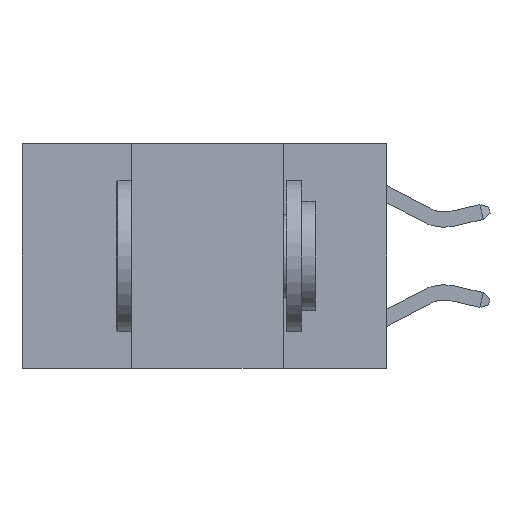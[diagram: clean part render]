
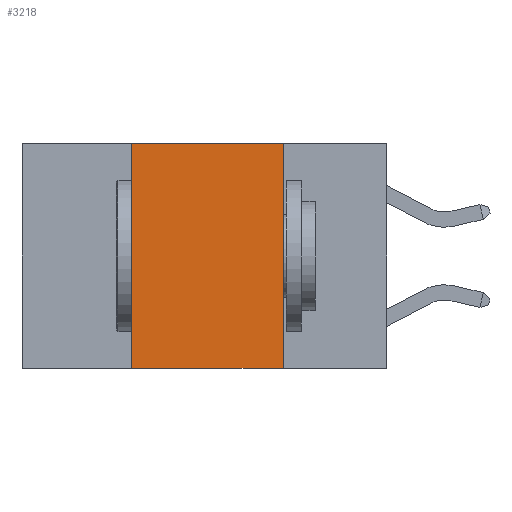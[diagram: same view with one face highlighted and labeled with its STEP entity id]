
A CAD part, left-side view. The second image highlights one B-rep face of the part: STEP entity #3218.
In plain terms, the highlighted planar face has unit normal (-1, 0, 0).
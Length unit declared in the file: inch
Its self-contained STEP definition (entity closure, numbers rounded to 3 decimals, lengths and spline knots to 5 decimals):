
#52 = DIRECTION ( 'NONE',  ( 1., 0., 0. ) ) ;
#83 = CARTESIAN_POINT ( 'NONE',  ( 0., 0.42, -0.37 ) ) ;
#806 = VERTEX_POINT ( 'NONE', #83 ) ;
#929 = VERTEX_POINT ( 'NONE', #12667 ) ;
#1819 = ORIENTED_EDGE ( 'NONE', *, *, #6716, .F. ) ;
#2478 = ORIENTED_EDGE ( 'NONE', *, *, #9090, .T. ) ;
#2516 = CARTESIAN_POINT ( 'NONE',  ( 0., 0.6, 0. ) ) ;
#3015 = DIRECTION ( 'NONE',  ( 0., 0., -1. ) ) ;
#3218 = ADVANCED_FACE ( 'NONE', ( #7715 ), #7903, .F. ) ;
#4309 = AXIS2_PLACEMENT_3D ( 'NONE', #4913, #52, #5985 ) ;
#4599 = DIRECTION ( 'NONE',  ( 0., -1., 0. ) ) ;
#4606 = CARTESIAN_POINT ( 'NONE',  ( 0., 0.6, -0.37 ) ) ;
#4913 = CARTESIAN_POINT ( 'NONE',  ( 0., 0.6, 0. ) ) ;
#5049 = VERTEX_POINT ( 'NONE', #6504 ) ;
#5470 = VECTOR ( 'NONE', #7691, 39.37008 ) ;
#5887 = LINE ( 'NONE', #2516, #11035 ) ;
#5985 = DIRECTION ( 'NONE',  ( 0., 0., -1. ) ) ;
#6270 = EDGE_CURVE ( 'NONE', #806, #10207, #7948, .T. ) ;
#6504 = CARTESIAN_POINT ( 'NONE',  ( 0., 0.17, 0. ) ) ;
#6660 = EDGE_LOOP ( 'NONE', ( #1819, #7339, #13161, #2478 ) ) ;
#6716 = EDGE_CURVE ( 'NONE', #5049, #929, #9691, .T. ) ;
#7280 = CARTESIAN_POINT ( 'NONE',  ( 0., 0.42, 0. ) ) ;
#7284 = VECTOR ( 'NONE', #3015, 39.37008 ) ;
#7339 = ORIENTED_EDGE ( 'NONE', *, *, #12444, .F. ) ;
#7691 = DIRECTION ( 'NONE',  ( 0., -1., 0. ) ) ;
#7715 = FACE_OUTER_BOUND ( 'NONE', #6660, .T. ) ;
#7903 = PLANE ( 'NONE',  #4309 ) ;
#7948 = LINE ( 'NONE', #9508, #8585 ) ;
#8504 = LINE ( 'NONE', #4606, #5470 ) ;
#8585 = VECTOR ( 'NONE', #10575, 39.37008 ) ;
#9090 = EDGE_CURVE ( 'NONE', #806, #929, #8504, .T. ) ;
#9508 = CARTESIAN_POINT ( 'NONE',  ( 0., 0.42, 0. ) ) ;
#9691 = LINE ( 'NONE', #10195, #7284 ) ;
#10195 = CARTESIAN_POINT ( 'NONE',  ( 0., 0.17, 0. ) ) ;
#10207 = VERTEX_POINT ( 'NONE', #7280 ) ;
#10575 = DIRECTION ( 'NONE',  ( 0., 0., 1. ) ) ;
#11035 = VECTOR ( 'NONE', #4599, 39.37008 ) ;
#12444 = EDGE_CURVE ( 'NONE', #10207, #5049, #5887, .T. ) ;
#12667 = CARTESIAN_POINT ( 'NONE',  ( 0., 0.17, -0.37 ) ) ;
#13161 = ORIENTED_EDGE ( 'NONE', *, *, #6270, .F. ) ;
